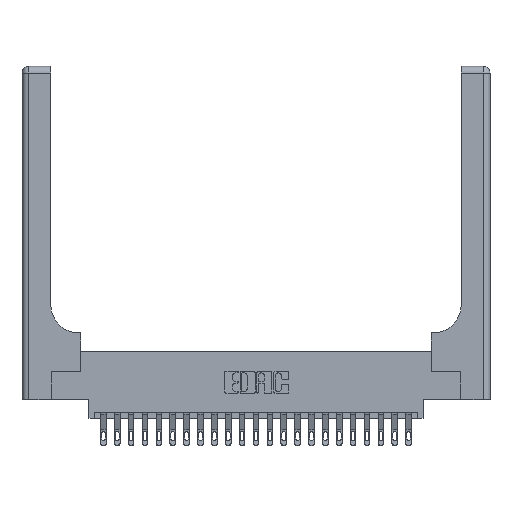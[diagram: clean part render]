
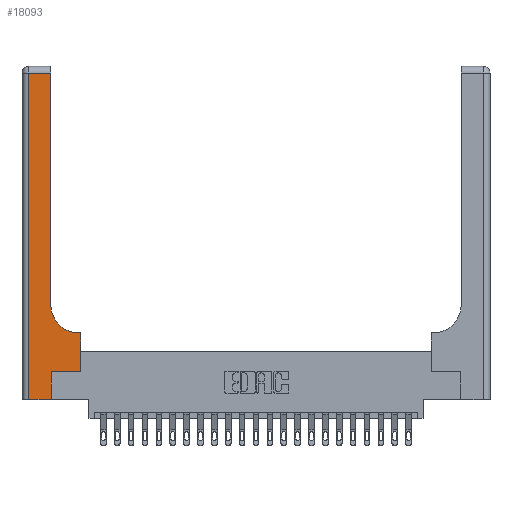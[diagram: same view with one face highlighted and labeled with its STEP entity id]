
A CAD part, top view. The second image highlights one B-rep face of the part: STEP entity #18093.
In plain terms, the highlighted planar face has unit normal (0, 0, 1).
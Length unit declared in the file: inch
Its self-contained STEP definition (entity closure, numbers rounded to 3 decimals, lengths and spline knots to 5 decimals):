
#75 = ORIENTED_EDGE ( 'NONE', *, *, #12708, .T. ) ;
#415 = VERTEX_POINT ( 'NONE', #22201 ) ;
#536 = DIRECTION ( 'NONE',  ( 1., 0., 0. ) ) ;
#675 = PLANE ( 'NONE',  #22678 ) ;
#676 = LINE ( 'NONE', #11864, #22282 ) ;
#710 = DIRECTION ( 'NONE',  ( 0., 1., 0. ) ) ;
#1453 = ORIENTED_EDGE ( 'NONE', *, *, #7413, .T. ) ;
#1597 = DIRECTION ( 'NONE',  ( -1., 0., 0. ) ) ;
#1951 = VERTEX_POINT ( 'NONE', #15715 ) ;
#2011 = ORIENTED_EDGE ( 'NONE', *, *, #10288, .T. ) ;
#2129 = ORIENTED_EDGE ( 'NONE', *, *, #11152, .T. ) ;
#2980 = LINE ( 'NONE', #13382, #17351 ) ;
#3739 = CARTESIAN_POINT ( 'NONE',  ( 0.06, 2.94, 0.37 ) ) ;
#4029 = CARTESIAN_POINT ( 'NONE',  ( 0.26, 0.85, 0.37 ) ) ;
#4043 = ORIENTED_EDGE ( 'NONE', *, *, #22948, .T. ) ;
#4154 = ORIENTED_EDGE ( 'NONE', *, *, #8822, .T. ) ;
#4493 = CARTESIAN_POINT ( 'NONE',  ( 0., 0., 0.37 ) ) ;
#5263 = CARTESIAN_POINT ( 'NONE',  ( 0.26, 0.6, 0.37 ) ) ;
#5425 = EDGE_CURVE ( 'NONE', #6308, #20268, #12580, .T. ) ;
#5823 = LINE ( 'NONE', #7360, #11791 ) ;
#6148 = CARTESIAN_POINT ( 'NONE',  ( 0., 3., 0.37 ) ) ;
#6254 = CARTESIAN_POINT ( 'NONE',  ( 0.265, 0., 0.37 ) ) ;
#6308 = VERTEX_POINT ( 'NONE', #20748 ) ;
#6792 = VERTEX_POINT ( 'NONE', #13061 ) ;
#7046 = VECTOR ( 'NONE', #1597, 39.37008 ) ;
#7360 = CARTESIAN_POINT ( 'NONE',  ( 0.265, 0.25, 0.37 ) ) ;
#7413 = EDGE_CURVE ( 'NONE', #1951, #11982, #11135, .T. ) ;
#7607 = LINE ( 'NONE', #5263, #7046 ) ;
#7964 = CARTESIAN_POINT ( 'NONE',  ( 0.06, 3., 0.37 ) ) ;
#8140 = DIRECTION ( 'NONE',  ( 1., 0., 0. ) ) ;
#8622 = VECTOR ( 'NONE', #10307, 39.37008 ) ;
#8822 = EDGE_CURVE ( 'NONE', #20673, #6308, #7607, .T. ) ;
#9015 = DIRECTION ( 'NONE',  ( 0., 1., 0. ) ) ;
#9080 = CARTESIAN_POINT ( 'NONE',  ( 0.528, 0.6, 0.37 ) ) ;
#9194 = LINE ( 'NONE', #20955, #8622 ) ;
#9535 = VECTOR ( 'NONE', #11650, 39.37008 ) ;
#9792 = DIRECTION ( 'NONE',  ( 0., 0., -1. ) ) ;
#9985 = VECTOR ( 'NONE', #8140, 39.37008 ) ;
#10094 = ORIENTED_EDGE ( 'NONE', *, *, #18964, .T. ) ;
#10112 = ORIENTED_EDGE ( 'NONE', *, *, #5425, .T. ) ;
#10274 = VECTOR ( 'NONE', #9015, 39.37008 ) ;
#10288 = EDGE_CURVE ( 'NONE', #10667, #1951, #13751, .T. ) ;
#10307 = DIRECTION ( 'NONE',  ( 0., 1., 0. ) ) ;
#10667 = VERTEX_POINT ( 'NONE', #3739 ) ;
#10852 = LINE ( 'NONE', #12700, #10274 ) ;
#11135 = LINE ( 'NONE', #4493, #9985 ) ;
#11152 = EDGE_CURVE ( 'NONE', #12422, #415, #5823, .T. ) ;
#11162 = CARTESIAN_POINT ( 'NONE',  ( 0.265, 0.25, 0.37 ) ) ;
#11246 = FACE_OUTER_BOUND ( 'NONE', #12097, .T. ) ;
#11408 = DIRECTION ( 'NONE',  ( 0., 0., -1. ) ) ;
#11650 = DIRECTION ( 'NONE',  ( 0., -1., 0. ) ) ;
#11791 = VECTOR ( 'NONE', #16485, 39.37008 ) ;
#11864 = CARTESIAN_POINT ( 'NONE',  ( 0., 2.94, 0.37 ) ) ;
#11982 = VERTEX_POINT ( 'NONE', #6254 ) ;
#12097 = EDGE_LOOP ( 'NONE', ( #4043, #75, #2011, #1453, #22370, #2129, #10094, #4154, #10112 ) ) ;
#12422 = VERTEX_POINT ( 'NONE', #11162 ) ;
#12580 = CIRCLE ( 'NONE', #21638, 0.25 ) ;
#12700 = CARTESIAN_POINT ( 'NONE',  ( 0.265, 0., 0.37 ) ) ;
#12708 = EDGE_CURVE ( 'NONE', #6792, #10667, #676, .T. ) ;
#13061 = CARTESIAN_POINT ( 'NONE',  ( 0.26, 2.94, 0.37 ) ) ;
#13382 = CARTESIAN_POINT ( 'NONE',  ( 0.26, 3., 0.37 ) ) ;
#13618 = EDGE_CURVE ( 'NONE', #11982, #12422, #10852, .T. ) ;
#13751 = LINE ( 'NONE', #7964, #9535 ) ;
#15715 = CARTESIAN_POINT ( 'NONE',  ( 0.06, 0., 0.37 ) ) ;
#16485 = DIRECTION ( 'NONE',  ( 1., 0., 0. ) ) ;
#17351 = VECTOR ( 'NONE', #710, 39.37008 ) ;
#18093 = ADVANCED_FACE ( 'NONE', ( #11246 ), #675, .F. ) ;
#18964 = EDGE_CURVE ( 'NONE', #415, #20673, #9194, .T. ) ;
#20268 = VERTEX_POINT ( 'NONE', #4029 ) ;
#20673 = VERTEX_POINT ( 'NONE', #9080 ) ;
#20748 = CARTESIAN_POINT ( 'NONE',  ( 0.51, 0.6, 0.37 ) ) ;
#20955 = CARTESIAN_POINT ( 'NONE',  ( 0.528, 0.25, 0.37 ) ) ;
#21638 = AXIS2_PLACEMENT_3D ( 'NONE', #22027, #11408, #536 ) ;
#22027 = CARTESIAN_POINT ( 'NONE',  ( 0.51, 0.85, 0.37 ) ) ;
#22201 = CARTESIAN_POINT ( 'NONE',  ( 0.528, 0.25, 0.37 ) ) ;
#22247 = DIRECTION ( 'NONE',  ( -1., 0., 0. ) ) ;
#22282 = VECTOR ( 'NONE', #22461, 39.37008 ) ;
#22370 = ORIENTED_EDGE ( 'NONE', *, *, #13618, .T. ) ;
#22461 = DIRECTION ( 'NONE',  ( -1., 0., 0. ) ) ;
#22678 = AXIS2_PLACEMENT_3D ( 'NONE', #6148, #9792, #22247 ) ;
#22948 = EDGE_CURVE ( 'NONE', #20268, #6792, #2980, .T. ) ;
